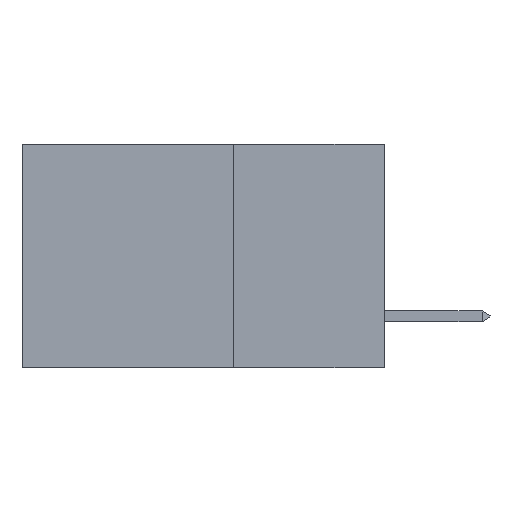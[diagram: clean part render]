
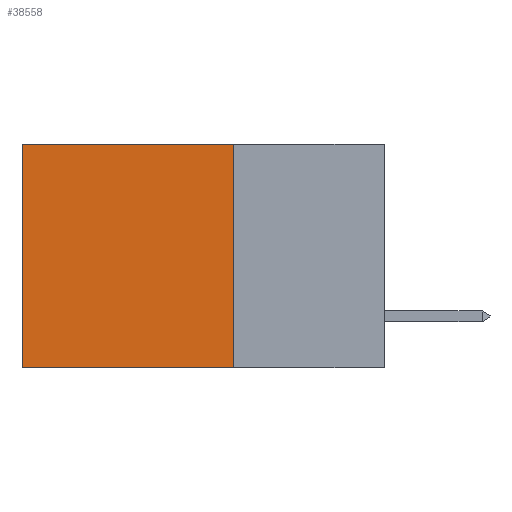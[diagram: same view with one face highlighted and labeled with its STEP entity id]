
A CAD part, left-side view. The second image highlights one B-rep face of the part: STEP entity #38558.
In plain terms, the highlighted planar face has unit normal (-1, 0, 0).
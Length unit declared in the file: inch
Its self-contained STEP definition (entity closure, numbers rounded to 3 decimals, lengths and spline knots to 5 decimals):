
#455 = ORIENTED_EDGE ( 'NONE', *, *, #2042, .T. ) ;
#496 = DIRECTION ( 'NONE',  ( 0., 0., -1. ) ) ;
#2042 = EDGE_CURVE ( 'NONE', #13597, #20677, #24171, .T. ) ;
#6222 = DIRECTION ( 'NONE',  ( 0., 0., -1. ) ) ;
#6678 = FACE_OUTER_BOUND ( 'NONE', #20849, .T. ) ;
#6917 = VECTOR ( 'NONE', #28095, 39.37008 ) ;
#7081 = CARTESIAN_POINT ( 'NONE',  ( 0.2875, 0.25, 0. ) ) ;
#8535 = EDGE_CURVE ( 'NONE', #31323, #15078, #19413, .T. ) ;
#9685 = CARTESIAN_POINT ( 'NONE',  ( 0.2875, 0.25, 0. ) ) ;
#11380 = CARTESIAN_POINT ( 'NONE',  ( 0.2875, 0.25, -0.37 ) ) ;
#11776 = CARTESIAN_POINT ( 'NONE',  ( 0.2875, 0.6, -0.37 ) ) ;
#12587 = CARTESIAN_POINT ( 'NONE',  ( 0.2875, 0.25, -0.37 ) ) ;
#13597 = VERTEX_POINT ( 'NONE', #24855 ) ;
#14075 = DIRECTION ( 'NONE',  ( 1., 0., 0. ) ) ;
#14681 = ORIENTED_EDGE ( 'NONE', *, *, #18410, .F. ) ;
#15078 = VERTEX_POINT ( 'NONE', #11776 ) ;
#16854 = PLANE ( 'NONE',  #43924 ) ;
#17260 = DIRECTION ( 'NONE',  ( 0., 0., -1. ) ) ;
#18410 = EDGE_CURVE ( 'NONE', #13597, #31323, #38556, .T. ) ;
#19121 = EDGE_CURVE ( 'NONE', #20677, #15078, #38676, .T. ) ;
#19413 = LINE ( 'NONE', #11380, #23036 ) ;
#20677 = VERTEX_POINT ( 'NONE', #34453 ) ;
#20849 = EDGE_LOOP ( 'NONE', ( #44444, #32778, #14681, #455 ) ) ;
#20872 = VECTOR ( 'NONE', #17260, 39.37008 ) ;
#23036 = VECTOR ( 'NONE', #39593, 39.37008 ) ;
#24171 = LINE ( 'NONE', #7081, #6917 ) ;
#24855 = CARTESIAN_POINT ( 'NONE',  ( 0.2875, 0.25, 0. ) ) ;
#25328 = VECTOR ( 'NONE', #496, 39.37008 ) ;
#28095 = DIRECTION ( 'NONE',  ( 0., 1., 0. ) ) ;
#31323 = VERTEX_POINT ( 'NONE', #12587 ) ;
#32778 = ORIENTED_EDGE ( 'NONE', *, *, #8535, .F. ) ;
#34453 = CARTESIAN_POINT ( 'NONE',  ( 0.2875, 0.6, 0. ) ) ;
#38556 = LINE ( 'NONE', #42258, #20872 ) ;
#38558 = ADVANCED_FACE ( 'NONE', ( #6678 ), #16854, .F. ) ;
#38676 = LINE ( 'NONE', #39127, #25328 ) ;
#39127 = CARTESIAN_POINT ( 'NONE',  ( 0.2875, 0.6, 0. ) ) ;
#39593 = DIRECTION ( 'NONE',  ( 0., 1., 0. ) ) ;
#42258 = CARTESIAN_POINT ( 'NONE',  ( 0.2875, 0.25, 0. ) ) ;
#43924 = AXIS2_PLACEMENT_3D ( 'NONE', #9685, #14075, #6222 ) ;
#44444 = ORIENTED_EDGE ( 'NONE', *, *, #19121, .T. ) ;
